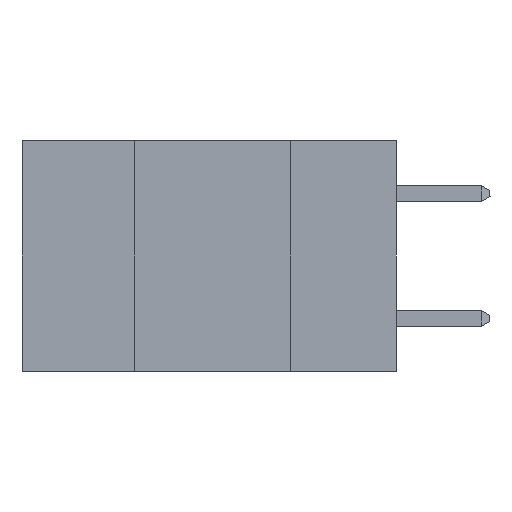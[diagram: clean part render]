
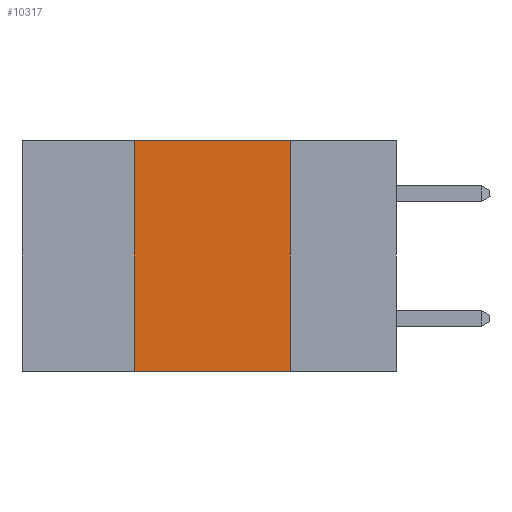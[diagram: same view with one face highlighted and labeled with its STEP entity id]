
A CAD part, left-side view. The second image highlights one B-rep face of the part: STEP entity #10317.
In plain terms, the highlighted planar face has unit normal (-1, 0, 0).
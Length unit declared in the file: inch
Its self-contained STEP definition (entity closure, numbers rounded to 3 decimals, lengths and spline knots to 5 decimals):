
#238 = ORIENTED_EDGE ( 'NONE', *, *, #17051, .F. ) ;
#1456 = CARTESIAN_POINT ( 'NONE',  ( 0., 0.6, 0. ) ) ;
#2424 = CARTESIAN_POINT ( 'NONE',  ( 0., 0.17, -0.37 ) ) ;
#3246 = DIRECTION ( 'NONE',  ( 1., 0., 0. ) ) ;
#4561 = LINE ( 'NONE', #5451, #13951 ) ;
#4844 = LINE ( 'NONE', #12847, #13119 ) ;
#5451 = CARTESIAN_POINT ( 'NONE',  ( 0., 0.17, 0. ) ) ;
#5481 = CARTESIAN_POINT ( 'NONE',  ( 0., 0.6, 0. ) ) ;
#7285 = VERTEX_POINT ( 'NONE', #2424 ) ;
#9695 = ORIENTED_EDGE ( 'NONE', *, *, #16161, .F. ) ;
#10317 = ADVANCED_FACE ( 'NONE', ( #18026 ), #22649, .F. ) ;
#11194 = DIRECTION ( 'NONE',  ( 0., 0., 1. ) ) ;
#12847 = CARTESIAN_POINT ( 'NONE',  ( 0., 0.42, 0. ) ) ;
#12992 = CARTESIAN_POINT ( 'NONE',  ( 0., 0.6, -0.37 ) ) ;
#13119 = VECTOR ( 'NONE', #11194, 39.37008 ) ;
#13812 = ORIENTED_EDGE ( 'NONE', *, *, #18520, .F. ) ;
#13951 = VECTOR ( 'NONE', #17811, 39.37008 ) ;
#14109 = VECTOR ( 'NONE', #14781, 39.37008 ) ;
#14357 = DIRECTION ( 'NONE',  ( 0., -1., 0. ) ) ;
#14781 = DIRECTION ( 'NONE',  ( 0., -1., 0. ) ) ;
#14821 = VERTEX_POINT ( 'NONE', #20630 ) ;
#14934 = ORIENTED_EDGE ( 'NONE', *, *, #20924, .T. ) ;
#15224 = LINE ( 'NONE', #12992, #14109 ) ;
#15390 = EDGE_LOOP ( 'NONE', ( #13812, #238, #9695, #14934 ) ) ;
#15631 = DIRECTION ( 'NONE',  ( 0., 0., -1. ) ) ;
#16161 = EDGE_CURVE ( 'NONE', #16240, #14821, #4844, .T. ) ;
#16240 = VERTEX_POINT ( 'NONE', #21989 ) ;
#16693 = CARTESIAN_POINT ( 'NONE',  ( 0., 0.17, 0. ) ) ;
#17051 = EDGE_CURVE ( 'NONE', #14821, #21416, #21955, .T. ) ;
#17250 = VECTOR ( 'NONE', #14357, 39.37008 ) ;
#17811 = DIRECTION ( 'NONE',  ( 0., 0., -1. ) ) ;
#18026 = FACE_OUTER_BOUND ( 'NONE', #15390, .T. ) ;
#18520 = EDGE_CURVE ( 'NONE', #21416, #7285, #4561, .T. ) ;
#20630 = CARTESIAN_POINT ( 'NONE',  ( 0., 0.42, 0. ) ) ;
#20924 = EDGE_CURVE ( 'NONE', #16240, #7285, #15224, .T. ) ;
#21416 = VERTEX_POINT ( 'NONE', #16693 ) ;
#21955 = LINE ( 'NONE', #5481, #17250 ) ;
#21989 = CARTESIAN_POINT ( 'NONE',  ( 0., 0.42, -0.37 ) ) ;
#22424 = AXIS2_PLACEMENT_3D ( 'NONE', #1456, #3246, #15631 ) ;
#22649 = PLANE ( 'NONE',  #22424 ) ;
